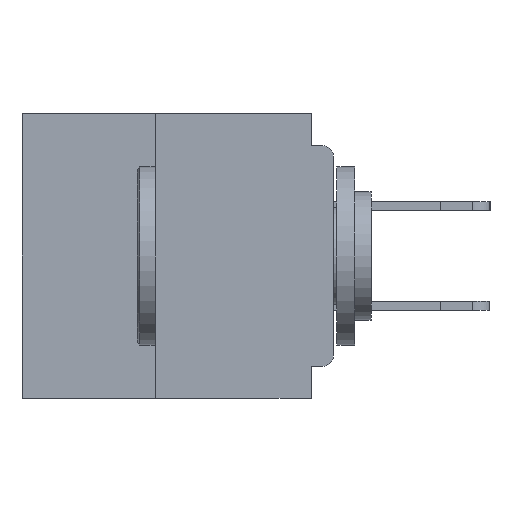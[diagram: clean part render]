
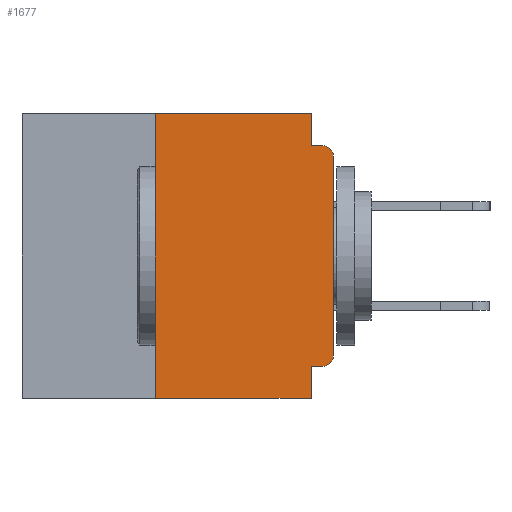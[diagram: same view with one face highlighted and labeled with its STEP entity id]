
A CAD part, left-side view. The second image highlights one B-rep face of the part: STEP entity #1677.
In plain terms, the highlighted planar face has unit normal (-1, 0, 0).
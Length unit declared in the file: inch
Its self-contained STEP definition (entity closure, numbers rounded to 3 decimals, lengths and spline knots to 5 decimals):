
#6 = DIRECTION ( 'NONE',  ( 0., -1., 0. ) ) ;
#72 = DIRECTION ( 'NONE',  ( 0., -1., 0. ) ) ;
#1677 = ADVANCED_FACE ( 'NONE', ( #2595 ), #23059, .F. ) ;
#1948 = DIRECTION ( 'NONE',  ( -1., 0., 0. ) ) ;
#2519 = ORIENTED_EDGE ( 'NONE', *, *, #7053, .F. ) ;
#2595 = FACE_OUTER_BOUND ( 'NONE', #23300, .T. ) ;
#3366 = CARTESIAN_POINT ( 'NONE',  ( 0., 0., -0.045 ) ) ;
#5023 = LINE ( 'NONE', #32769, #29413 ) ;
#6313 = VERTEX_POINT ( 'NONE', #19734 ) ;
#6385 = VECTOR ( 'NONE', #32413, 39.37008 ) ;
#6521 = CARTESIAN_POINT ( 'NONE',  ( 0., 0., 0. ) ) ;
#6939 = CARTESIAN_POINT ( 'NONE',  ( 0., 0.015, -0.355 ) ) ;
#7053 = EDGE_CURVE ( 'NONE', #36079, #10525, #31706, .T. ) ;
#7277 = VECTOR ( 'NONE', #28757, 39.37008 ) ;
#8229 = AXIS2_PLACEMENT_3D ( 'NONE', #21045, #1948, #24234 ) ;
#8343 = CARTESIAN_POINT ( 'NONE',  ( 0., 0.015, -0.06 ) ) ;
#9376 = DIRECTION ( 'NONE',  ( 0., 1., 0. ) ) ;
#10063 = CARTESIAN_POINT ( 'NONE',  ( 0., 0., -0.34 ) ) ;
#10433 = DIRECTION ( 'NONE',  ( 0., 0., 1. ) ) ;
#10525 = VERTEX_POINT ( 'NONE', #33806 ) ;
#11150 = ORIENTED_EDGE ( 'NONE', *, *, #14194, .T. ) ;
#11546 = DIRECTION ( 'NONE',  ( 0., 0., -1. ) ) ;
#12032 = VECTOR ( 'NONE', #9376, 39.37008 ) ;
#12091 = CARTESIAN_POINT ( 'NONE',  ( 0., 0., -0.06 ) ) ;
#13263 = LINE ( 'NONE', #33335, #20734 ) ;
#13441 = ORIENTED_EDGE ( 'NONE', *, *, #29279, .F. ) ;
#13524 = ORIENTED_EDGE ( 'NONE', *, *, #27579, .F. ) ;
#14194 = EDGE_CURVE ( 'NONE', #40306, #27416, #34948, .T. ) ;
#14228 = VERTEX_POINT ( 'NONE', #30747 ) ;
#14467 = EDGE_CURVE ( 'NONE', #24050, #36079, #32467, .T. ) ;
#14919 = ORIENTED_EDGE ( 'NONE', *, *, #15677, .F. ) ;
#15578 = ORIENTED_EDGE ( 'NONE', *, *, #19223, .T. ) ;
#15677 = EDGE_CURVE ( 'NONE', #40306, #14228, #37289, .T. ) ;
#15778 = LINE ( 'NONE', #3366, #31663 ) ;
#18043 = VECTOR ( 'NONE', #6, 39.37008 ) ;
#19223 = EDGE_CURVE ( 'NONE', #38263, #30072, #37290, .T. ) ;
#19734 = CARTESIAN_POINT ( 'NONE',  ( 0., 0.25, -0.4 ) ) ;
#20734 = VECTOR ( 'NONE', #36463, 39.37008 ) ;
#21045 = CARTESIAN_POINT ( 'NONE',  ( 0., 0.015, -0.34 ) ) ;
#22539 = CARTESIAN_POINT ( 'NONE',  ( 0., 0.437, 0. ) ) ;
#23059 = PLANE ( 'NONE',  #29520 ) ;
#23200 = CARTESIAN_POINT ( 'NONE',  ( 0., 0.031, -0.4 ) ) ;
#23300 = EDGE_LOOP ( 'NONE', ( #27419, #15578, #13441, #2519, #36895, #13524, #41102, #34535, #14919, #11150 ) ) ;
#24050 = VERTEX_POINT ( 'NONE', #38144 ) ;
#24234 = DIRECTION ( 'NONE',  ( 0., 0., -1. ) ) ;
#24847 = EDGE_CURVE ( 'NONE', #27416, #38263, #32576, .T. ) ;
#25516 = LINE ( 'NONE', #31892, #18043 ) ;
#26008 = DIRECTION ( 'NONE',  ( 0., 0., -1. ) ) ;
#26841 = EDGE_CURVE ( 'NONE', #6313, #28097, #25516, .T. ) ;
#27416 = VERTEX_POINT ( 'NONE', #10063 ) ;
#27419 = ORIENTED_EDGE ( 'NONE', *, *, #24847, .T. ) ;
#27579 = EDGE_CURVE ( 'NONE', #6313, #24050, #5023, .T. ) ;
#27790 = CARTESIAN_POINT ( 'NONE',  ( 0., 0.437, 0. ) ) ;
#28097 = VERTEX_POINT ( 'NONE', #23200 ) ;
#28757 = DIRECTION ( 'NONE',  ( 0., 0., 1. ) ) ;
#28823 = DIRECTION ( 'NONE',  ( 0., -1., 0. ) ) ;
#29279 = EDGE_CURVE ( 'NONE', #10525, #30072, #15778, .T. ) ;
#29413 = VECTOR ( 'NONE', #10433, 39.37008 ) ;
#29414 = CARTESIAN_POINT ( 'NONE',  ( 0., 0.031, 0. ) ) ;
#29520 = AXIS2_PLACEMENT_3D ( 'NONE', #27790, #30048, #26008 ) ;
#29568 = EDGE_CURVE ( 'NONE', #14228, #28097, #13263, .T. ) ;
#30048 = DIRECTION ( 'NONE',  ( 1., 0., 0. ) ) ;
#30072 = VERTEX_POINT ( 'NONE', #39061 ) ;
#30576 = DIRECTION ( 'NONE',  ( -1., 0., 0. ) ) ;
#30747 = CARTESIAN_POINT ( 'NONE',  ( 0., 0.031, -0.355 ) ) ;
#31586 = CARTESIAN_POINT ( 'NONE',  ( 0., 0.031, 0. ) ) ;
#31663 = VECTOR ( 'NONE', #28823, 39.37008 ) ;
#31706 = LINE ( 'NONE', #29414, #6385 ) ;
#31758 = AXIS2_PLACEMENT_3D ( 'NONE', #8343, #30576, #11546 ) ;
#31892 = CARTESIAN_POINT ( 'NONE',  ( 0., 0.437, -0.4 ) ) ;
#32413 = DIRECTION ( 'NONE',  ( 0., 0., -1. ) ) ;
#32467 = LINE ( 'NONE', #22539, #40835 ) ;
#32576 = LINE ( 'NONE', #6521, #7277 ) ;
#32769 = CARTESIAN_POINT ( 'NONE',  ( 0., 0.25, -0.4 ) ) ;
#33335 = CARTESIAN_POINT ( 'NONE',  ( 0., 0.031, -0.4 ) ) ;
#33806 = CARTESIAN_POINT ( 'NONE',  ( 0., 0.031, -0.045 ) ) ;
#34535 = ORIENTED_EDGE ( 'NONE', *, *, #29568, .F. ) ;
#34617 = CARTESIAN_POINT ( 'NONE',  ( 0., 0., -0.355 ) ) ;
#34948 = CIRCLE ( 'NONE', #8229, 0.015 ) ;
#36079 = VERTEX_POINT ( 'NONE', #31586 ) ;
#36463 = DIRECTION ( 'NONE',  ( 0., 0., -1. ) ) ;
#36895 = ORIENTED_EDGE ( 'NONE', *, *, #14467, .F. ) ;
#37289 = LINE ( 'NONE', #34617, #12032 ) ;
#37290 = CIRCLE ( 'NONE', #31758, 0.015 ) ;
#38144 = CARTESIAN_POINT ( 'NONE',  ( 0., 0.25, 0. ) ) ;
#38263 = VERTEX_POINT ( 'NONE', #12091 ) ;
#39061 = CARTESIAN_POINT ( 'NONE',  ( 0., 0.015, -0.045 ) ) ;
#40306 = VERTEX_POINT ( 'NONE', #6939 ) ;
#40835 = VECTOR ( 'NONE', #72, 39.37008 ) ;
#41102 = ORIENTED_EDGE ( 'NONE', *, *, #26841, .T. ) ;
